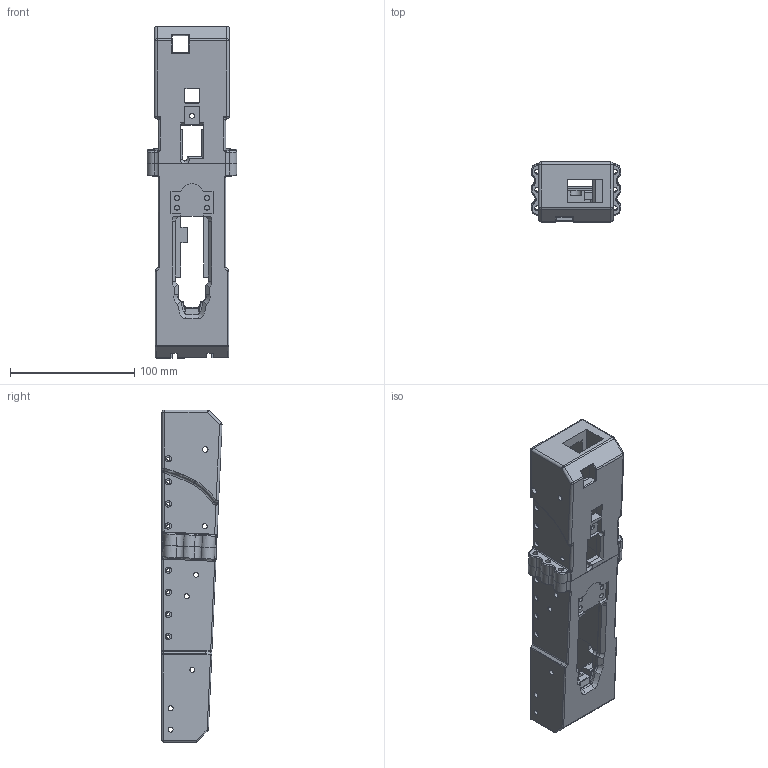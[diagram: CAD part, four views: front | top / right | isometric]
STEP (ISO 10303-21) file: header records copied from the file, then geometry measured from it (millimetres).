
FILE_DESCRIPTION(/* description */ (''),/* implementation_level */ '2;1');
FILE_NAME(/* name */ 'Plastikov v0.9 Assembly.stp',/* time_stamp */ '2019-12-22T15:45:07-06:00',/* author */ ('johne'),/* organization */ (''),/* preprocessor_version */ 'ST-DEVELOPER v18',/* originating_system */ 'Autodesk Inventor 2020',/* authorisation */ '');
FILE_SCHEMA (('AUTOMOTIVE_DESIGN { 1 0 10303 214 3 1 1 }'));
Products named in the file (5): Assembly1; Plastikov v0.9 Front Receiver; Plastikov v0.9 Left Rail; Plastikov v0.9 Rear Receiver; Plastikov v0.9 Right Rail
Assembly tree (4 placements, depth 2):
  Assembly1
    Plastikov v0.9 Front Receiver
    Plastikov v0.9 Left Rail
    Plastikov v0.9 Rear Receiver
    Plastikov v0.9 Right Rail
Bounding box: 72.2 x 48.28 x 267 mm (x, y, z)
Volume: 346318.3 mm3; surface area: 101469.4 mm2
Topology: 4 solids, 4 shells, 610 faces, 1612 edges, 1021 vertices
Faces by surface type: plane 259, cylinder 209, bspline 65, torus 43, sphere 27, cone 7
Full cylindrical faces by diameter (mm): 2.5 x32, 3 x4, 3.12 x4, 4 x29, 4.05 x1, 4.5 x2, 5.08 x16
Entity records: 21445 total; most frequent: CARTESIAN_POINT 5793, DIRECTION 3259, ORIENTED_EDGE 3192, EDGE_CURVE 1596, AXIS2_PLACEMENT_3D 1203, VERTEX_POINT 1021, LINE 853, VECTOR 853
